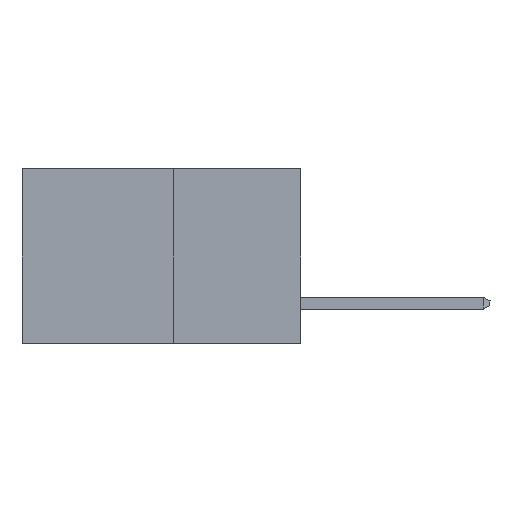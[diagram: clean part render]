
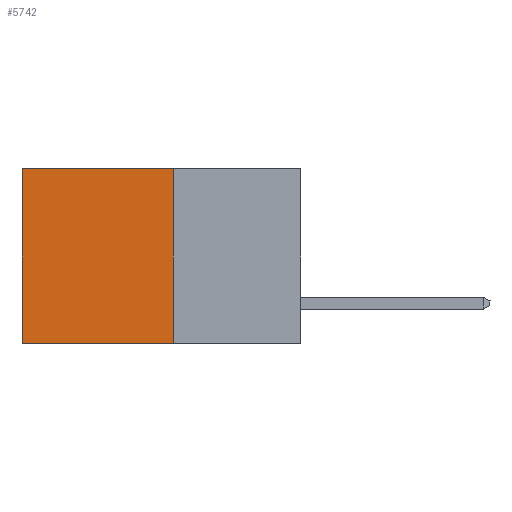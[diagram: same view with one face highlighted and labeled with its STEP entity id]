
A CAD part, left-side view. The second image highlights one B-rep face of the part: STEP entity #5742.
In plain terms, the highlighted planar face has unit normal (-1, 0, 0).
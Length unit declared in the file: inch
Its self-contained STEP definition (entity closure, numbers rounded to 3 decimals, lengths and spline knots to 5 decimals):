
#454 = VERTEX_POINT ( 'NONE', #5650 ) ;
#487 = EDGE_CURVE ( 'NONE', #5062, #454, #2699, .T. ) ;
#621 = DIRECTION ( 'NONE',  ( 0., 0., -1. ) ) ;
#1578 = ORIENTED_EDGE ( 'NONE', *, *, #487, .T. ) ;
#2016 = DIRECTION ( 'NONE',  ( 0., 0., -1. ) ) ;
#2068 = VERTEX_POINT ( 'NONE', #7097 ) ;
#2099 = LINE ( 'NONE', #9327, #8737 ) ;
#2218 = ORIENTED_EDGE ( 'NONE', *, *, #11180, .F. ) ;
#2293 = ORIENTED_EDGE ( 'NONE', *, *, #9278, .F. ) ;
#2699 = LINE ( 'NONE', #5444, #4745 ) ;
#2756 = CARTESIAN_POINT ( 'NONE',  ( 0.277, 0.27, 0. ) ) ;
#3078 = CARTESIAN_POINT ( 'NONE',  ( 0.277, 0.59, 0. ) ) ;
#3196 = VERTEX_POINT ( 'NONE', #8818 ) ;
#3642 = DIRECTION ( 'NONE',  ( 0., 1., 0. ) ) ;
#3819 = LINE ( 'NONE', #2756, #10313 ) ;
#4135 = CARTESIAN_POINT ( 'NONE',  ( 0.277, 0.27, -0.37 ) ) ;
#4136 = VECTOR ( 'NONE', #2016, 39.37008 ) ;
#4211 = PLANE ( 'NONE',  #10663 ) ;
#4745 = VECTOR ( 'NONE', #5441, 39.37008 ) ;
#5062 = VERTEX_POINT ( 'NONE', #3078 ) ;
#5441 = DIRECTION ( 'NONE',  ( 0., 0., -1. ) ) ;
#5444 = CARTESIAN_POINT ( 'NONE',  ( 0.277, 0.59, -0.37 ) ) ;
#5650 = CARTESIAN_POINT ( 'NONE',  ( 0.277, 0.59, -0.37 ) ) ;
#5742 = ADVANCED_FACE ( 'NONE', ( #6433 ), #4211, .F. ) ;
#5926 = DIRECTION ( 'NONE',  ( 1., 0., 0. ) ) ;
#6080 = ORIENTED_EDGE ( 'NONE', *, *, #8865, .T. ) ;
#6433 = FACE_OUTER_BOUND ( 'NONE', #7489, .T. ) ;
#7097 = CARTESIAN_POINT ( 'NONE',  ( 0.277, 0.27, 0. ) ) ;
#7489 = EDGE_LOOP ( 'NONE', ( #1578, #2293, #2218, #6080 ) ) ;
#8709 = LINE ( 'NONE', #9753, #4136 ) ;
#8737 = VECTOR ( 'NONE', #10130, 39.37008 ) ;
#8818 = CARTESIAN_POINT ( 'NONE',  ( 0.277, 0.27, -0.37 ) ) ;
#8865 = EDGE_CURVE ( 'NONE', #2068, #5062, #3819, .T. ) ;
#9278 = EDGE_CURVE ( 'NONE', #3196, #454, #2099, .T. ) ;
#9327 = CARTESIAN_POINT ( 'NONE',  ( 0.277, 0.27, -0.37 ) ) ;
#9753 = CARTESIAN_POINT ( 'NONE',  ( 0.277, 0.27, -0.37 ) ) ;
#10130 = DIRECTION ( 'NONE',  ( 0., 1., 0. ) ) ;
#10313 = VECTOR ( 'NONE', #3642, 39.37008 ) ;
#10663 = AXIS2_PLACEMENT_3D ( 'NONE', #4135, #5926, #621 ) ;
#11180 = EDGE_CURVE ( 'NONE', #2068, #3196, #8709, .T. ) ;
